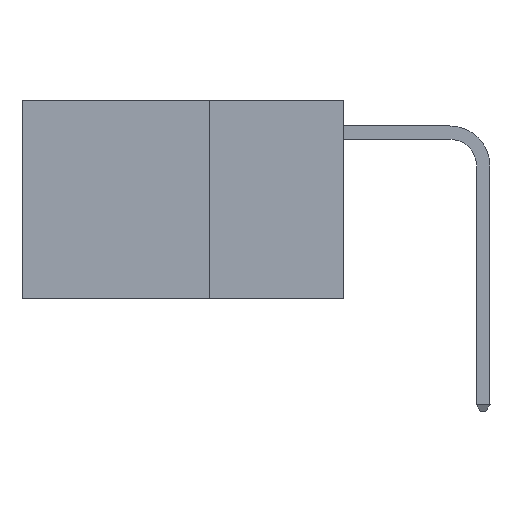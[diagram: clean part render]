
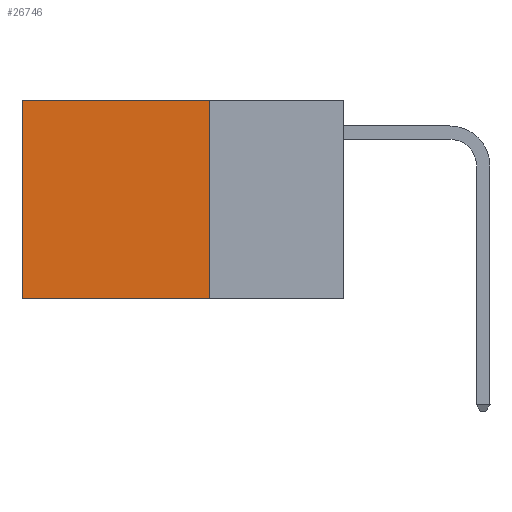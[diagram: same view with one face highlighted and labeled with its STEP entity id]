
A CAD part, left-side view. The second image highlights one B-rep face of the part: STEP entity #26746.
In plain terms, the highlighted planar face has unit normal (-1, 0, 0).
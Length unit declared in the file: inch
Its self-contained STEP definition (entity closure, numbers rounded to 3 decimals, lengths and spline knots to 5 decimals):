
#644 = DIRECTION ( 'NONE',  ( 0., 1., 0. ) ) ;
#907 = VECTOR ( 'NONE', #7900, 39.37008 ) ;
#1108 = VECTOR ( 'NONE', #6676, 39.37008 ) ;
#1800 = LINE ( 'NONE', #13308, #1108 ) ;
#2224 = EDGE_LOOP ( 'NONE', ( #22670, #26842, #8420, #21186 ) ) ;
#4992 = EDGE_CURVE ( 'NONE', #6259, #10549, #21515, .T. ) ;
#5670 = VECTOR ( 'NONE', #27202, 39.37008 ) ;
#6259 = VERTEX_POINT ( 'NONE', #23977 ) ;
#6676 = DIRECTION ( 'NONE',  ( 0., 0., -1. ) ) ;
#7338 = VERTEX_POINT ( 'NONE', #21152 ) ;
#7900 = DIRECTION ( 'NONE',  ( 0., 0., -1. ) ) ;
#7947 = CARTESIAN_POINT ( 'NONE',  ( 0.2625, 0.6, -0.37 ) ) ;
#8420 = ORIENTED_EDGE ( 'NONE', *, *, #20797, .F. ) ;
#10549 = VERTEX_POINT ( 'NONE', #24030 ) ;
#10731 = DIRECTION ( 'NONE',  ( 0., 0., -1. ) ) ;
#13308 = CARTESIAN_POINT ( 'NONE',  ( 0.2625, 0.25, 0. ) ) ;
#14883 = EDGE_CURVE ( 'NONE', #7338, #17298, #22973, .T. ) ;
#15363 = FACE_OUTER_BOUND ( 'NONE', #2224, .T. ) ;
#15871 = VECTOR ( 'NONE', #644, 39.37008 ) ;
#17298 = VERTEX_POINT ( 'NONE', #7947 ) ;
#17856 = LINE ( 'NONE', #20893, #907 ) ;
#18550 = EDGE_CURVE ( 'NONE', #10549, #17298, #17856, .T. ) ;
#19043 = CARTESIAN_POINT ( 'NONE',  ( 0.2625, 0.25, -0.37 ) ) ;
#20322 = CARTESIAN_POINT ( 'NONE',  ( 0.2625, 0.25, 0. ) ) ;
#20797 = EDGE_CURVE ( 'NONE', #6259, #7338, #1800, .T. ) ;
#20893 = CARTESIAN_POINT ( 'NONE',  ( 0.2625, 0.6, 0. ) ) ;
#21152 = CARTESIAN_POINT ( 'NONE',  ( 0.2625, 0.25, -0.37 ) ) ;
#21186 = ORIENTED_EDGE ( 'NONE', *, *, #4992, .T. ) ;
#21280 = AXIS2_PLACEMENT_3D ( 'NONE', #27708, #23549, #10731 ) ;
#21443 = PLANE ( 'NONE',  #21280 ) ;
#21515 = LINE ( 'NONE', #20322, #15871 ) ;
#22670 = ORIENTED_EDGE ( 'NONE', *, *, #18550, .T. ) ;
#22973 = LINE ( 'NONE', #19043, #5670 ) ;
#23549 = DIRECTION ( 'NONE',  ( 1., 0., 0. ) ) ;
#23977 = CARTESIAN_POINT ( 'NONE',  ( 0.2625, 0.25, 0. ) ) ;
#24030 = CARTESIAN_POINT ( 'NONE',  ( 0.2625, 0.6, 0. ) ) ;
#26746 = ADVANCED_FACE ( 'NONE', ( #15363 ), #21443, .F. ) ;
#26842 = ORIENTED_EDGE ( 'NONE', *, *, #14883, .F. ) ;
#27202 = DIRECTION ( 'NONE',  ( 0., 1., 0. ) ) ;
#27708 = CARTESIAN_POINT ( 'NONE',  ( 0.2625, 0.25, 0. ) ) ;
